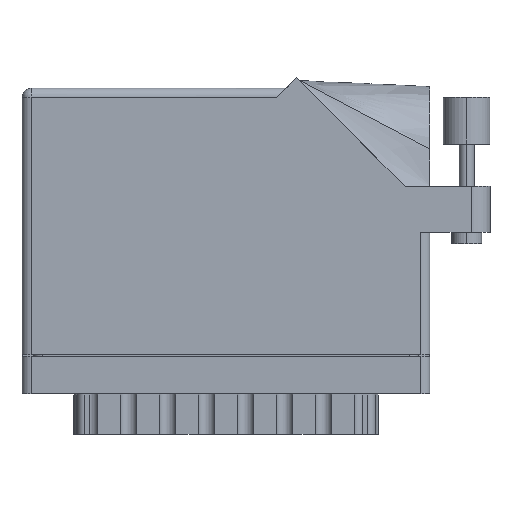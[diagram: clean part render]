
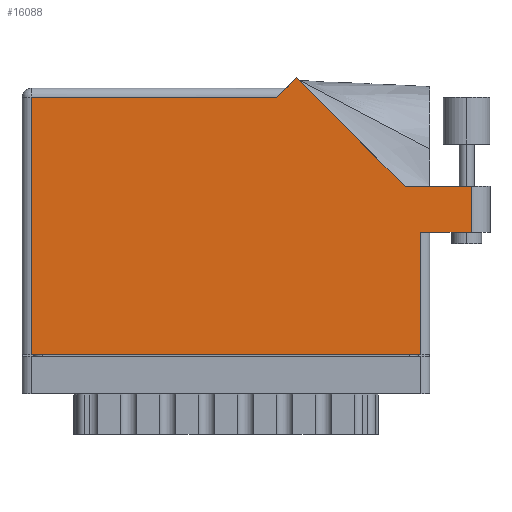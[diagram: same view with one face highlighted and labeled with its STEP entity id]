
A CAD part, front view. The second image highlights one B-rep face of the part: STEP entity #16088.
In plain terms, the highlighted face is planar.
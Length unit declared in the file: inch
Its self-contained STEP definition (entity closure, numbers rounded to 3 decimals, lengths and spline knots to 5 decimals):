
#710 = VECTOR ( 'NONE', #20787, 39.37008 ) ;
#1135 = CARTESIAN_POINT ( 'NONE',  ( 0.062, 0., 0. ) ) ;
#2342 = VECTOR ( 'NONE', #33469, 39.37008 ) ;
#2666 = CARTESIAN_POINT ( 'NONE',  ( 2.55242, 1.122, 0. ) ) ;
#3471 = DIRECTION ( 'NONE',  ( 0., 1., 0. ) ) ;
#3883 = EDGE_CURVE ( 'NONE', #64913, #10925, #57646, .T. ) ;
#4522 = VECTOR ( 'NONE', #42622, 39.37008 ) ;
#4525 = ORIENTED_EDGE ( 'NONE', *, *, #32573, .T. ) ;
#7306 = CARTESIAN_POINT ( 'NONE',  ( 0., 1.713, 0. ) ) ;
#7705 = VERTEX_POINT ( 'NONE', #15941 ) ;
#7976 = VERTEX_POINT ( 'NONE', #28891 ) ;
#9892 = ORIENTED_EDGE ( 'NONE', *, *, #44950, .T. ) ;
#10206 = EDGE_CURVE ( 'NONE', #7976, #7705, #66153, .T. ) ;
#10925 = VERTEX_POINT ( 'NONE', #23813 ) ;
#11029 = LINE ( 'NONE', #35182, #4522 ) ;
#13038 = VECTOR ( 'NONE', #29076, 39.37008 ) ;
#14691 = CARTESIAN_POINT ( 'NONE',  ( 0., 0., 0. ) ) ;
#15109 = PLANE ( 'NONE',  #17445 ) ;
#15870 = CARTESIAN_POINT ( 'NONE',  ( 2.656, 0.815, 0. ) ) ;
#15941 = CARTESIAN_POINT ( 'NONE',  ( 1.696, 1.713, 0. ) ) ;
#16088 = ADVANCED_FACE ( 'NONE', ( #51755 ), #15109, .F. ) ;
#16617 = VECTOR ( 'NONE', #54003, 39.37008 ) ;
#17445 = AXIS2_PLACEMENT_3D ( 'NONE', #36225, #20319, #19875 ) ;
#17812 = LINE ( 'NONE', #7306, #2342 ) ;
#19875 = DIRECTION ( 'NONE',  ( -1., 0., 0. ) ) ;
#20319 = DIRECTION ( 'NONE',  ( 0., 0., -1. ) ) ;
#20787 = DIRECTION ( 'NONE',  ( 1., 0., 0. ) ) ;
#21343 = ORIENTED_EDGE ( 'NONE', *, *, #55340, .T. ) ;
#23813 = CARTESIAN_POINT ( 'NONE',  ( 2.656, 0., 0. ) ) ;
#24725 = DIRECTION ( 'NONE',  ( -0.707, -0.707, 0. ) ) ;
#26878 = LINE ( 'NONE', #2666, #13038 ) ;
#28492 = EDGE_CURVE ( 'NONE', #37536, #64913, #11029, .T. ) ;
#28891 = CARTESIAN_POINT ( 'NONE',  ( 1.82871, 1.84571, 0. ) ) ;
#29076 = DIRECTION ( 'NONE',  ( -0.707, 0.707, 0. ) ) ;
#29979 = EDGE_CURVE ( 'NONE', #10925, #51247, #33717, .T. ) ;
#30515 = EDGE_LOOP ( 'NONE', ( #21343, #9892, #4525, #30757, #40475, #42580, #52797, #52598, #36332 ) ) ;
#30536 = CARTESIAN_POINT ( 'NONE',  ( 2.993, 0.815, 0. ) ) ;
#30757 = ORIENTED_EDGE ( 'NONE', *, *, #32255, .T. ) ;
#31509 = DIRECTION ( 'NONE',  ( -1., 0., 0. ) ) ;
#32003 = VECTOR ( 'NONE', #24725, 39.37008 ) ;
#32255 = EDGE_CURVE ( 'NONE', #36039, #7976, #26878, .T. ) ;
#32573 = EDGE_CURVE ( 'NONE', #40628, #36039, #67478, .T. ) ;
#32982 = CARTESIAN_POINT ( 'NONE',  ( 2.55242, 1.122, 0. ) ) ;
#33224 = EDGE_CURVE ( 'NONE', #7705, #37536, #17812, .T. ) ;
#33469 = DIRECTION ( 'NONE',  ( -1., 0., 0. ) ) ;
#33717 = LINE ( 'NONE', #39642, #39402 ) ;
#34012 = CARTESIAN_POINT ( 'NONE',  ( 2.993, 1.122, 0. ) ) ;
#34926 = CARTESIAN_POINT ( 'NONE',  ( 1.758, 1.775, 0. ) ) ;
#35182 = CARTESIAN_POINT ( 'NONE',  ( 0.062, 0., 0. ) ) ;
#35305 = DIRECTION ( 'NONE',  ( 1., 0., 0. ) ) ;
#36039 = VERTEX_POINT ( 'NONE', #32982 ) ;
#36225 = CARTESIAN_POINT ( 'NONE',  ( 0., 1.775, 0. ) ) ;
#36332 = ORIENTED_EDGE ( 'NONE', *, *, #29979, .T. ) ;
#37536 = VERTEX_POINT ( 'NONE', #42457 ) ;
#37888 = CARTESIAN_POINT ( 'NONE',  ( 3.118, 1.122, 0. ) ) ;
#39402 = VECTOR ( 'NONE', #3471, 39.37008 ) ;
#39642 = CARTESIAN_POINT ( 'NONE',  ( 2.656, 0.815, 0. ) ) ;
#40475 = ORIENTED_EDGE ( 'NONE', *, *, #10206, .T. ) ;
#40628 = VERTEX_POINT ( 'NONE', #60001 ) ;
#42457 = CARTESIAN_POINT ( 'NONE',  ( 0.062, 1.713, 0. ) ) ;
#42580 = ORIENTED_EDGE ( 'NONE', *, *, #33224, .T. ) ;
#42622 = DIRECTION ( 'NONE',  ( 0., -1., 0. ) ) ;
#44950 = EDGE_CURVE ( 'NONE', #64693, #40628, #60497, .T. ) ;
#51247 = VERTEX_POINT ( 'NONE', #15870 ) ;
#51755 = FACE_OUTER_BOUND ( 'NONE', #30515, .T. ) ;
#52598 = ORIENTED_EDGE ( 'NONE', *, *, #3883, .T. ) ;
#52797 = ORIENTED_EDGE ( 'NONE', *, *, #28492, .T. ) ;
#54003 = DIRECTION ( 'NONE',  ( 0., 1., 0. ) ) ;
#54075 = VECTOR ( 'NONE', #35305, 39.37008 ) ;
#55340 = EDGE_CURVE ( 'NONE', #51247, #64693, #61411, .T. ) ;
#55504 = CARTESIAN_POINT ( 'NONE',  ( 2.718, 0.815, 0. ) ) ;
#57646 = LINE ( 'NONE', #14691, #710 ) ;
#60001 = CARTESIAN_POINT ( 'NONE',  ( 2.993, 1.122, 0. ) ) ;
#60497 = LINE ( 'NONE', #34012, #16617 ) ;
#61411 = LINE ( 'NONE', #55504, #54075 ) ;
#64693 = VERTEX_POINT ( 'NONE', #30536 ) ;
#64913 = VERTEX_POINT ( 'NONE', #1135 ) ;
#65064 = VECTOR ( 'NONE', #31509, 39.37008 ) ;
#66153 = LINE ( 'NONE', #34926, #32003 ) ;
#67478 = LINE ( 'NONE', #37888, #65064 ) ;
